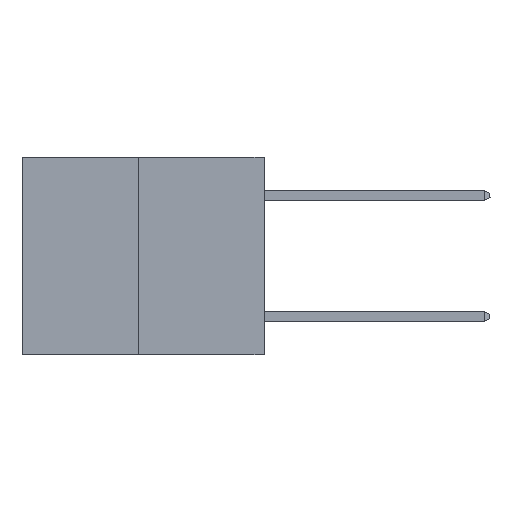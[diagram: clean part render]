
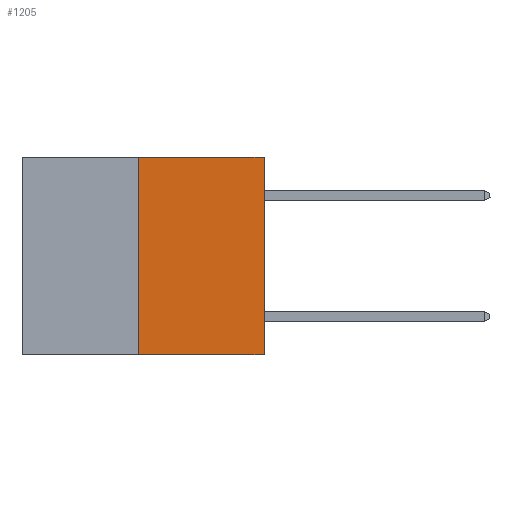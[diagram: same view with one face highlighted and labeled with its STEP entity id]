
A CAD part, left-side view. The second image highlights one B-rep face of the part: STEP entity #1205.
In plain terms, the highlighted planar face has unit normal (-1, 0, 0).
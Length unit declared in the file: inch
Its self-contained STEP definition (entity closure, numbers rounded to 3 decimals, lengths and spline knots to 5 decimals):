
#547 = ORIENTED_EDGE ( 'NONE', *, *, #8183, .F. ) ;
#1205 = ADVANCED_FACE ( 'NONE', ( #12759 ), #22130, .F. ) ;
#1367 = ORIENTED_EDGE ( 'NONE', *, *, #11487, .T. ) ;
#1747 = DIRECTION ( 'NONE',  ( 1., 0., 0. ) ) ;
#3003 = VERTEX_POINT ( 'NONE', #6834 ) ;
#3297 = DIRECTION ( 'NONE',  ( 0., -1., 0. ) ) ;
#3522 = AXIS2_PLACEMENT_3D ( 'NONE', #18345, #1747, #9139 ) ;
#4201 = VECTOR ( 'NONE', #3297, 39.37008 ) ;
#5346 = LINE ( 'NONE', #6003, #12898 ) ;
#5485 = CARTESIAN_POINT ( 'NONE',  ( 0., 0.6, -0.49 ) ) ;
#6003 = CARTESIAN_POINT ( 'NONE',  ( 0., 0.6, 0. ) ) ;
#6226 = VERTEX_POINT ( 'NONE', #17044 ) ;
#6834 = CARTESIAN_POINT ( 'NONE',  ( 0., 0.312, -0.49 ) ) ;
#7846 = EDGE_LOOP ( 'NONE', ( #547, #1367, #24101, #9810 ) ) ;
#7993 = DIRECTION ( 'NONE',  ( 0., 0., 1. ) ) ;
#8183 = EDGE_CURVE ( 'NONE', #3003, #19277, #8542, .T. ) ;
#8542 = LINE ( 'NONE', #22191, #14639 ) ;
#9139 = DIRECTION ( 'NONE',  ( 0., 0., -1. ) ) ;
#9712 = LINE ( 'NONE', #5485, #4201 ) ;
#9810 = ORIENTED_EDGE ( 'NONE', *, *, #11801, .F. ) ;
#11080 = CARTESIAN_POINT ( 'NONE',  ( 0., 0.312, 0. ) ) ;
#11487 = EDGE_CURVE ( 'NONE', #3003, #13945, #9712, .T. ) ;
#11588 = DIRECTION ( 'NONE',  ( 0., -1., 0. ) ) ;
#11711 = CARTESIAN_POINT ( 'NONE',  ( 0., 0., 0. ) ) ;
#11733 = VECTOR ( 'NONE', #7993, 39.37008 ) ;
#11801 = EDGE_CURVE ( 'NONE', #19277, #6226, #5346, .T. ) ;
#12759 = FACE_OUTER_BOUND ( 'NONE', #7846, .T. ) ;
#12898 = VECTOR ( 'NONE', #11588, 39.37008 ) ;
#13361 = CARTESIAN_POINT ( 'NONE',  ( 0., 0., -0.49 ) ) ;
#13945 = VERTEX_POINT ( 'NONE', #13361 ) ;
#14639 = VECTOR ( 'NONE', #20567, 39.37008 ) ;
#17044 = CARTESIAN_POINT ( 'NONE',  ( 0., 0., 0. ) ) ;
#18345 = CARTESIAN_POINT ( 'NONE',  ( 0., 0.6, 0. ) ) ;
#19277 = VERTEX_POINT ( 'NONE', #11080 ) ;
#19569 = EDGE_CURVE ( 'NONE', #13945, #6226, #21709, .T. ) ;
#20567 = DIRECTION ( 'NONE',  ( 0., 0., 1. ) ) ;
#21709 = LINE ( 'NONE', #11711, #11733 ) ;
#22130 = PLANE ( 'NONE',  #3522 ) ;
#22191 = CARTESIAN_POINT ( 'NONE',  ( 0., 0.312, -0.49 ) ) ;
#24101 = ORIENTED_EDGE ( 'NONE', *, *, #19569, .T. ) ;
